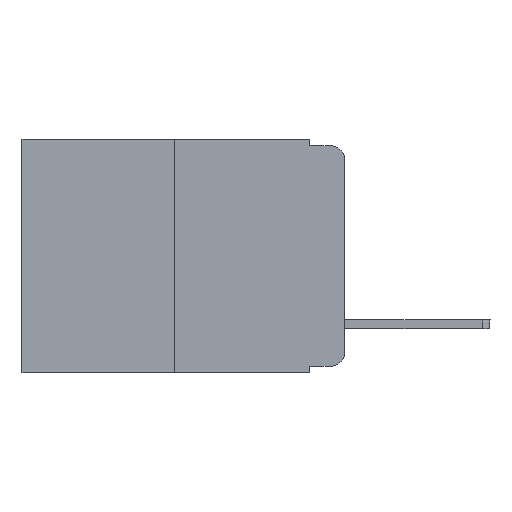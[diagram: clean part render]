
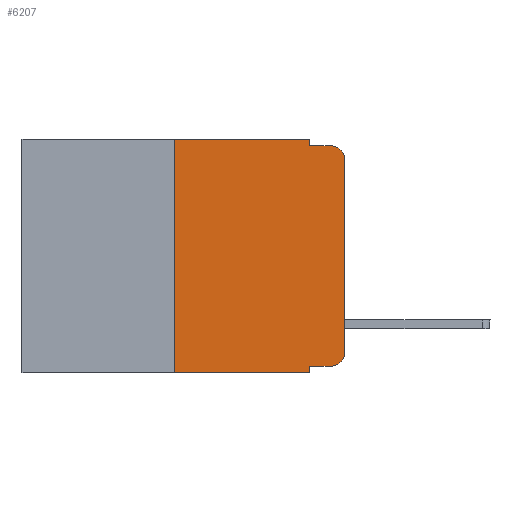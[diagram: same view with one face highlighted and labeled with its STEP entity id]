
A CAD part, left-side view. The second image highlights one B-rep face of the part: STEP entity #6207.
In plain terms, the highlighted planar face has unit normal (-1, 0, 0).
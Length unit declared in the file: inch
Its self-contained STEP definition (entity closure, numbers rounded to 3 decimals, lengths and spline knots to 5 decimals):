
#107 = VERTEX_POINT ( 'NONE', #16584 ) ;
#272 = VECTOR ( 'NONE', #9915, 39.37008 ) ;
#419 = LINE ( 'NONE', #509, #8332 ) ;
#509 = CARTESIAN_POINT ( 'NONE',  ( 0., 0., 0. ) ) ;
#555 = CARTESIAN_POINT ( 'NONE',  ( 0., 0.051, -0.01 ) ) ;
#614 = VECTOR ( 'NONE', #15715, 39.37008 ) ;
#698 = CARTESIAN_POINT ( 'NONE',  ( 0., 0.473, 0. ) ) ;
#1455 = EDGE_CURVE ( 'NONE', #3878, #9327, #5729, .T. ) ;
#1864 = ORIENTED_EDGE ( 'NONE', *, *, #17512, .F. ) ;
#2010 = VERTEX_POINT ( 'NONE', #2018 ) ;
#2018 = CARTESIAN_POINT ( 'NONE',  ( 0., 0.051, -0.01 ) ) ;
#2217 = CARTESIAN_POINT ( 'NONE',  ( 0., 0.02, -0.333 ) ) ;
#2311 = CARTESIAN_POINT ( 'NONE',  ( 0., 0.051, 0. ) ) ;
#2911 = CARTESIAN_POINT ( 'NONE',  ( 0., 0., -0.03 ) ) ;
#3575 = FACE_OUTER_BOUND ( 'NONE', #15958, .T. ) ;
#3592 = EDGE_CURVE ( 'NONE', #107, #3878, #11624, .T. ) ;
#3598 = CIRCLE ( 'NONE', #7567, 0.02 ) ;
#3878 = VERTEX_POINT ( 'NONE', #6896 ) ;
#3879 = CARTESIAN_POINT ( 'NONE',  ( 0., 0., -0.313 ) ) ;
#4246 = EDGE_CURVE ( 'NONE', #16908, #4698, #419, .T. ) ;
#4482 = LINE ( 'NONE', #8746, #272 ) ;
#4698 = VERTEX_POINT ( 'NONE', #2911 ) ;
#4939 = CARTESIAN_POINT ( 'NONE',  ( 0., 0.02, -0.01 ) ) ;
#5097 = ORIENTED_EDGE ( 'NONE', *, *, #8596, .T. ) ;
#5148 = CARTESIAN_POINT ( 'NONE',  ( 0., 0.051, 0. ) ) ;
#5336 = CARTESIAN_POINT ( 'NONE',  ( 0., 0.02, -0.03 ) ) ;
#5708 = VECTOR ( 'NONE', #13376, 39.37008 ) ;
#5729 = LINE ( 'NONE', #5986, #8479 ) ;
#5863 = ORIENTED_EDGE ( 'NONE', *, *, #6623, .F. ) ;
#5986 = CARTESIAN_POINT ( 'NONE',  ( 0., 0.473, 0. ) ) ;
#6207 = ADVANCED_FACE ( 'NONE', ( #3575 ), #17027, .F. ) ;
#6537 = CIRCLE ( 'NONE', #7657, 0.02 ) ;
#6613 = VERTEX_POINT ( 'NONE', #2217 ) ;
#6623 = EDGE_CURVE ( 'NONE', #9327, #2010, #14418, .T. ) ;
#6896 = CARTESIAN_POINT ( 'NONE',  ( 0., 0.25, 0. ) ) ;
#7120 = VERTEX_POINT ( 'NONE', #8717 ) ;
#7292 = DIRECTION ( 'NONE',  ( 0., 0., 1. ) ) ;
#7351 = CARTESIAN_POINT ( 'NONE',  ( 0., 0.25, 0. ) ) ;
#7386 = VECTOR ( 'NONE', #15587, 39.37008 ) ;
#7487 = DIRECTION ( 'NONE',  ( 1., 0., 0. ) ) ;
#7567 = AXIS2_PLACEMENT_3D ( 'NONE', #5336, #10937, #10669 ) ;
#7594 = LINE ( 'NONE', #555, #10171 ) ;
#7657 = AXIS2_PLACEMENT_3D ( 'NONE', #15460, #11292, #8527 ) ;
#7945 = CARTESIAN_POINT ( 'NONE',  ( 0., 0.473, -0.343 ) ) ;
#8332 = VECTOR ( 'NONE', #7292, 39.37008 ) ;
#8479 = VECTOR ( 'NONE', #9908, 39.37008 ) ;
#8527 = DIRECTION ( 'NONE',  ( 0., 0., -1. ) ) ;
#8596 = EDGE_CURVE ( 'NONE', #6613, #16908, #6537, .T. ) ;
#8717 = CARTESIAN_POINT ( 'NONE',  ( 0., 0.051, -0.333 ) ) ;
#8746 = CARTESIAN_POINT ( 'NONE',  ( 0., 0.051, 0. ) ) ;
#8769 = ORIENTED_EDGE ( 'NONE', *, *, #4246, .T. ) ;
#9220 = ORIENTED_EDGE ( 'NONE', *, *, #1455, .F. ) ;
#9243 = ORIENTED_EDGE ( 'NONE', *, *, #3592, .F. ) ;
#9309 = ORIENTED_EDGE ( 'NONE', *, *, #13115, .F. ) ;
#9327 = VERTEX_POINT ( 'NONE', #5148 ) ;
#9821 = DIRECTION ( 'NONE',  ( 0., -1., 0. ) ) ;
#9908 = DIRECTION ( 'NONE',  ( 0., -1., 0. ) ) ;
#9915 = DIRECTION ( 'NONE',  ( 0., 0., -1. ) ) ;
#9925 = EDGE_CURVE ( 'NONE', #7120, #6613, #16585, .T. ) ;
#10171 = VECTOR ( 'NONE', #11519, 39.37008 ) ;
#10669 = DIRECTION ( 'NONE',  ( 0., 0., -1. ) ) ;
#10710 = LINE ( 'NONE', #7945, #5708 ) ;
#10907 = VECTOR ( 'NONE', #9821, 39.37008 ) ;
#10937 = DIRECTION ( 'NONE',  ( -1., 0., 0. ) ) ;
#10975 = CARTESIAN_POINT ( 'NONE',  ( 0., 0.051, -0.343 ) ) ;
#11292 = DIRECTION ( 'NONE',  ( -1., 0., 0. ) ) ;
#11519 = DIRECTION ( 'NONE',  ( 0., -1., 0. ) ) ;
#11624 = LINE ( 'NONE', #7351, #614 ) ;
#12750 = CARTESIAN_POINT ( 'NONE',  ( 0., 0.051, -0.333 ) ) ;
#13070 = VERTEX_POINT ( 'NONE', #10975 ) ;
#13098 = EDGE_CURVE ( 'NONE', #107, #13070, #10710, .T. ) ;
#13115 = EDGE_CURVE ( 'NONE', #7120, #13070, #4482, .T. ) ;
#13182 = ORIENTED_EDGE ( 'NONE', *, *, #13098, .T. ) ;
#13203 = ORIENTED_EDGE ( 'NONE', *, *, #16575, .T. ) ;
#13376 = DIRECTION ( 'NONE',  ( 0., -1., 0. ) ) ;
#13443 = ORIENTED_EDGE ( 'NONE', *, *, #9925, .T. ) ;
#13879 = AXIS2_PLACEMENT_3D ( 'NONE', #698, #7487, #17111 ) ;
#14418 = LINE ( 'NONE', #2311, #7386 ) ;
#15460 = CARTESIAN_POINT ( 'NONE',  ( 0., 0.02, -0.313 ) ) ;
#15587 = DIRECTION ( 'NONE',  ( 0., 0., -1. ) ) ;
#15715 = DIRECTION ( 'NONE',  ( 0., 0., 1. ) ) ;
#15958 = EDGE_LOOP ( 'NONE', ( #8769, #13203, #1864, #5863, #9220, #9243, #13182, #9309, #13443, #5097 ) ) ;
#16575 = EDGE_CURVE ( 'NONE', #4698, #17571, #3598, .T. ) ;
#16584 = CARTESIAN_POINT ( 'NONE',  ( 0., 0.25, -0.343 ) ) ;
#16585 = LINE ( 'NONE', #12750, #10907 ) ;
#16908 = VERTEX_POINT ( 'NONE', #3879 ) ;
#17027 = PLANE ( 'NONE',  #13879 ) ;
#17111 = DIRECTION ( 'NONE',  ( 0., 0., -1. ) ) ;
#17512 = EDGE_CURVE ( 'NONE', #2010, #17571, #7594, .T. ) ;
#17571 = VERTEX_POINT ( 'NONE', #4939 ) ;
